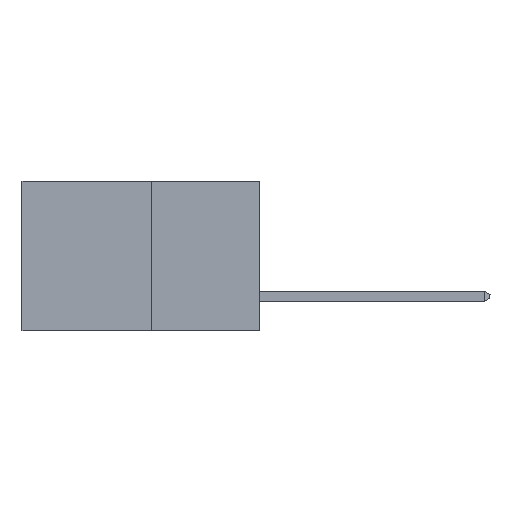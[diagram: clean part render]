
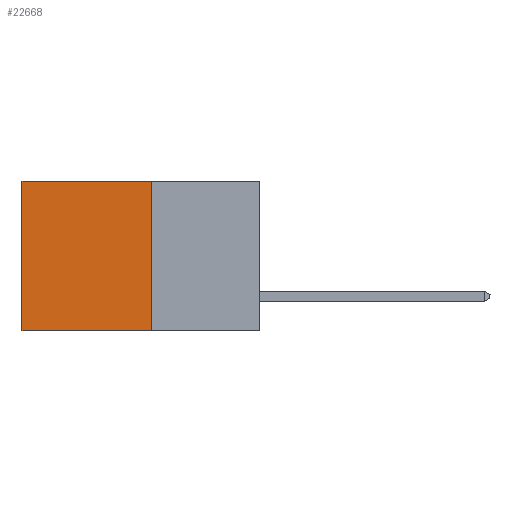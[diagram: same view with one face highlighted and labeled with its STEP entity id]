
A CAD part, left-side view. The second image highlights one B-rep face of the part: STEP entity #22668.
In plain terms, the highlighted planar face has unit normal (-1, 0, 0).
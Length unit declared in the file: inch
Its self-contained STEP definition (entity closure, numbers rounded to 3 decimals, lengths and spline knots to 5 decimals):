
#1538 = VECTOR ( 'NONE', #10280, 39.37008 ) ;
#2243 = DIRECTION ( 'NONE',  ( 1., 0., 0. ) ) ;
#3470 = VERTEX_POINT ( 'NONE', #30252 ) ;
#3607 = VECTOR ( 'NONE', #21247, 39.37008 ) ;
#4477 = DIRECTION ( 'NONE',  ( 0., 1., 0. ) ) ;
#4918 = CARTESIAN_POINT ( 'NONE',  ( 0.277, 0.59, -0.37 ) ) ;
#5390 = VECTOR ( 'NONE', #19635, 39.37008 ) ;
#5945 = EDGE_CURVE ( 'NONE', #10637, #23250, #27200, .T. ) ;
#10280 = DIRECTION ( 'NONE',  ( 0., 1., 0. ) ) ;
#10637 = VERTEX_POINT ( 'NONE', #19598 ) ;
#10717 = ORIENTED_EDGE ( 'NONE', *, *, #30151, .F. ) ;
#11678 = LINE ( 'NONE', #21854, #5390 ) ;
#12183 = FACE_OUTER_BOUND ( 'NONE', #14432, .T. ) ;
#13874 = CARTESIAN_POINT ( 'NONE',  ( 0.277, 0.27, -0.37 ) ) ;
#14432 = EDGE_LOOP ( 'NONE', ( #26227, #26034, #10717, #18872 ) ) ;
#16383 = LINE ( 'NONE', #13874, #22536 ) ;
#18656 = DIRECTION ( 'NONE',  ( 0., 0., -1. ) ) ;
#18693 = EDGE_CURVE ( 'NONE', #3470, #21823, #16383, .T. ) ;
#18872 = ORIENTED_EDGE ( 'NONE', *, *, #5945, .T. ) ;
#19598 = CARTESIAN_POINT ( 'NONE',  ( 0.277, 0.27, 0. ) ) ;
#19635 = DIRECTION ( 'NONE',  ( 0., 0., -1. ) ) ;
#21247 = DIRECTION ( 'NONE',  ( 0., 0., -1. ) ) ;
#21823 = VERTEX_POINT ( 'NONE', #27344 ) ;
#21854 = CARTESIAN_POINT ( 'NONE',  ( 0.277, 0.27, -0.37 ) ) ;
#22536 = VECTOR ( 'NONE', #4477, 39.37008 ) ;
#22668 = ADVANCED_FACE ( 'NONE', ( #12183 ), #25576, .F. ) ;
#23250 = VERTEX_POINT ( 'NONE', #23385 ) ;
#23385 = CARTESIAN_POINT ( 'NONE',  ( 0.277, 0.59, 0. ) ) ;
#24196 = AXIS2_PLACEMENT_3D ( 'NONE', #27895, #2243, #18656 ) ;
#25576 = PLANE ( 'NONE',  #24196 ) ;
#26034 = ORIENTED_EDGE ( 'NONE', *, *, #18693, .F. ) ;
#26227 = ORIENTED_EDGE ( 'NONE', *, *, #26241, .T. ) ;
#26241 = EDGE_CURVE ( 'NONE', #23250, #21823, #27709, .T. ) ;
#26551 = CARTESIAN_POINT ( 'NONE',  ( 0.277, 0.27, 0. ) ) ;
#27200 = LINE ( 'NONE', #26551, #1538 ) ;
#27344 = CARTESIAN_POINT ( 'NONE',  ( 0.277, 0.59, -0.37 ) ) ;
#27709 = LINE ( 'NONE', #4918, #3607 ) ;
#27895 = CARTESIAN_POINT ( 'NONE',  ( 0.277, 0.27, -0.37 ) ) ;
#30151 = EDGE_CURVE ( 'NONE', #10637, #3470, #11678, .T. ) ;
#30252 = CARTESIAN_POINT ( 'NONE',  ( 0.277, 0.27, -0.37 ) ) ;
